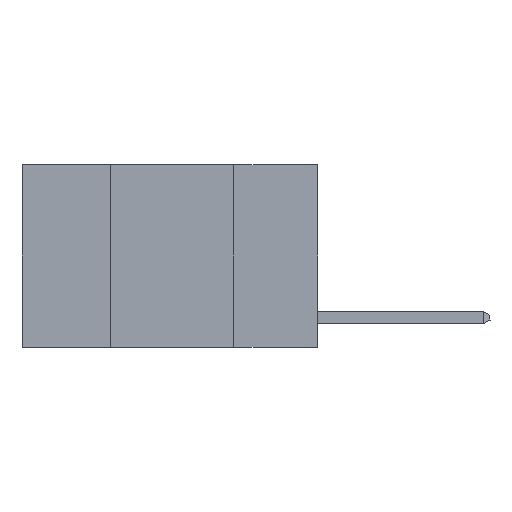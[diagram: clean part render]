
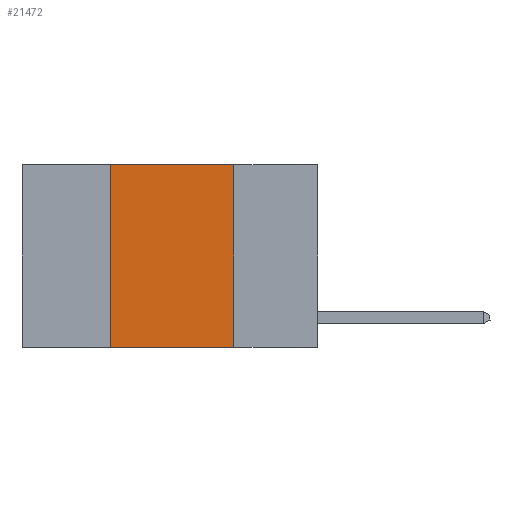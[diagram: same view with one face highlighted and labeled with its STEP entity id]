
A CAD part, left-side view. The second image highlights one B-rep face of the part: STEP entity #21472.
In plain terms, the highlighted planar face has unit normal (-1, 0, 0).
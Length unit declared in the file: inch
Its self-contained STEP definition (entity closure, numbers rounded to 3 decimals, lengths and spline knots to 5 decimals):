
#238 = PLANE ( 'NONE',  #10347 ) ;
#980 = CARTESIAN_POINT ( 'NONE',  ( 0., 0.6, 0. ) ) ;
#3103 = LINE ( 'NONE', #980, #15601 ) ;
#3474 = CARTESIAN_POINT ( 'NONE',  ( 0., 0.17, -0.37 ) ) ;
#5331 = DIRECTION ( 'NONE',  ( 1., 0., 0. ) ) ;
#5645 = FACE_OUTER_BOUND ( 'NONE', #11611, .T. ) ;
#5806 = EDGE_CURVE ( 'NONE', #12398, #6419, #3103, .T. ) ;
#6419 = VERTEX_POINT ( 'NONE', #7768 ) ;
#7768 = CARTESIAN_POINT ( 'NONE',  ( 0., 0.17, 0. ) ) ;
#10188 = ORIENTED_EDGE ( 'NONE', *, *, #5806, .F. ) ;
#10332 = CARTESIAN_POINT ( 'NONE',  ( 0., 0.42, 0. ) ) ;
#10347 = AXIS2_PLACEMENT_3D ( 'NONE', #18777, #5331, #17169 ) ;
#11151 = DIRECTION ( 'NONE',  ( 0., -1., 0. ) ) ;
#11199 = LINE ( 'NONE', #21109, #15174 ) ;
#11456 = LINE ( 'NONE', #13518, #19849 ) ;
#11611 = EDGE_LOOP ( 'NONE', ( #14861, #10188, #12158, #12631 ) ) ;
#12158 = ORIENTED_EDGE ( 'NONE', *, *, #17999, .F. ) ;
#12398 = VERTEX_POINT ( 'NONE', #10332 ) ;
#12631 = ORIENTED_EDGE ( 'NONE', *, *, #12874, .T. ) ;
#12662 = EDGE_CURVE ( 'NONE', #6419, #13614, #11199, .T. ) ;
#12772 = DIRECTION ( 'NONE',  ( 0., 0., -1. ) ) ;
#12874 = EDGE_CURVE ( 'NONE', #13598, #13614, #11456, .T. ) ;
#13518 = CARTESIAN_POINT ( 'NONE',  ( 0., 0.6, -0.37 ) ) ;
#13598 = VERTEX_POINT ( 'NONE', #20373 ) ;
#13614 = VERTEX_POINT ( 'NONE', #3474 ) ;
#14861 = ORIENTED_EDGE ( 'NONE', *, *, #12662, .F. ) ;
#14923 = VECTOR ( 'NONE', #19191, 39.37008 ) ;
#15174 = VECTOR ( 'NONE', #12772, 39.37008 ) ;
#15235 = DIRECTION ( 'NONE',  ( 0., -1., 0. ) ) ;
#15601 = VECTOR ( 'NONE', #11151, 39.37008 ) ;
#17169 = DIRECTION ( 'NONE',  ( 0., 0., -1. ) ) ;
#17999 = EDGE_CURVE ( 'NONE', #13598, #12398, #19363, .T. ) ;
#18777 = CARTESIAN_POINT ( 'NONE',  ( 0., 0.6, 0. ) ) ;
#19123 = CARTESIAN_POINT ( 'NONE',  ( 0., 0.42, 0. ) ) ;
#19191 = DIRECTION ( 'NONE',  ( 0., 0., 1. ) ) ;
#19363 = LINE ( 'NONE', #19123, #14923 ) ;
#19849 = VECTOR ( 'NONE', #15235, 39.37008 ) ;
#20373 = CARTESIAN_POINT ( 'NONE',  ( 0., 0.42, -0.37 ) ) ;
#21109 = CARTESIAN_POINT ( 'NONE',  ( 0., 0.17, 0. ) ) ;
#21472 = ADVANCED_FACE ( 'NONE', ( #5645 ), #238, .F. ) ;
